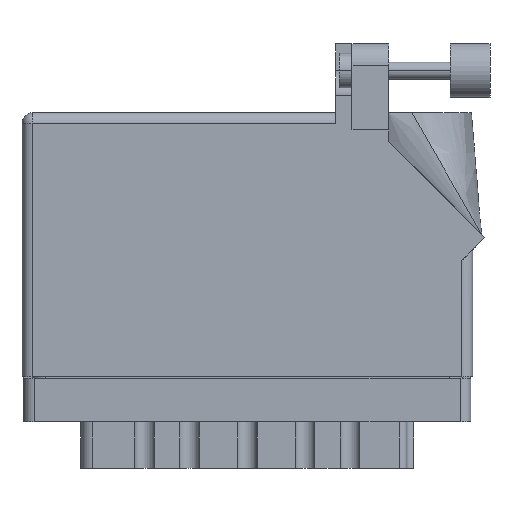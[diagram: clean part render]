
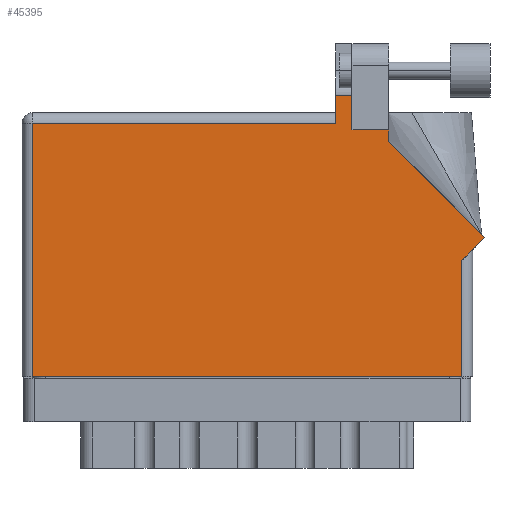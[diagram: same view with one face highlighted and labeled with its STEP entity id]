
A CAD part, front view. The second image highlights one B-rep face of the part: STEP entity #45395.
In plain terms, the highlighted face is planar.
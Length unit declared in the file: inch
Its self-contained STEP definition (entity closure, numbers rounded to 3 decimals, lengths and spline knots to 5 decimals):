
#1114 = CARTESIAN_POINT ( 'NONE',  ( 2.126, 1.43, 0. ) ) ;
#1149 = VERTEX_POINT ( 'NONE', #8238 ) ;
#3136 = VECTOR ( 'NONE', #6639, 39.37008 ) ;
#3262 = CARTESIAN_POINT ( 'NONE',  ( 2.55, 0., 0. ) ) ;
#3443 = ORIENTED_EDGE ( 'NONE', *, *, #29169, .T. ) ;
#3731 = DIRECTION ( 'NONE',  ( 0., 1., 0. ) ) ;
#4015 = CARTESIAN_POINT ( 'NONE',  ( 0., 1.468, 0. ) ) ;
#4046 = VERTEX_POINT ( 'NONE', #38259 ) ;
#4047 = LINE ( 'NONE', #37966, #14964 ) ;
#4328 = VERTEX_POINT ( 'NONE', #36645 ) ;
#4902 = CARTESIAN_POINT ( 'NONE',  ( 1.819, 1.53, 0. ) ) ;
#5037 = FACE_OUTER_BOUND ( 'NONE', #15050, .T. ) ;
#5993 = VERTEX_POINT ( 'NONE', #21692 ) ;
#6279 = DIRECTION ( 'NONE',  ( 0.707, 0.707, 0. ) ) ;
#6639 = DIRECTION ( 'NONE',  ( -1., 0., 0. ) ) ;
#6946 = VERTEX_POINT ( 'NONE', #3262 ) ;
#7095 = CARTESIAN_POINT ( 'NONE',  ( 1.913, 1.43, 0. ) ) ;
#7754 = LINE ( 'NONE', #4015, #37918 ) ;
#7974 = LINE ( 'NONE', #23871, #23864 ) ;
#8238 = CARTESIAN_POINT ( 'NONE',  ( 2.68271, 0.80771, 0. ) ) ;
#8385 = CARTESIAN_POINT ( 'NONE',  ( 2.55, 0.675, 0. ) ) ;
#9418 = ORIENTED_EDGE ( 'NONE', *, *, #36121, .T. ) ;
#9593 = CARTESIAN_POINT ( 'NONE',  ( 2.68271, 0.80771, 0. ) ) ;
#9613 = CARTESIAN_POINT ( 'NONE',  ( 0., 0., 0. ) ) ;
#10214 = CARTESIAN_POINT ( 'NONE',  ( 0.062, 0., 0. ) ) ;
#10884 = VECTOR ( 'NONE', #15582, 39.37008 ) ;
#12349 = EDGE_CURVE ( 'NONE', #29909, #5993, #34075, .T. ) ;
#12456 = ORIENTED_EDGE ( 'NONE', *, *, #20645, .T. ) ;
#12509 = EDGE_CURVE ( 'NONE', #32654, #39599, #7754, .T. ) ;
#13100 = DIRECTION ( 'NONE',  ( 1., 0., 0. ) ) ;
#14572 = DIRECTION ( 'NONE',  ( -1., 0., 0. ) ) ;
#14684 = CARTESIAN_POINT ( 'NONE',  ( 1.819, 1.468, 0. ) ) ;
#14956 = VERTEX_POINT ( 'NONE', #15863 ) ;
#14964 = VECTOR ( 'NONE', #6279, 39.37008 ) ;
#15033 = VERTEX_POINT ( 'NONE', #8385 ) ;
#15050 = EDGE_LOOP ( 'NONE', ( #31628, #37266, #26577, #32310, #3443, #44332, #22404, #15284, #9418, #12456, #29070 ) ) ;
#15099 = LINE ( 'NONE', #9613, #18404 ) ;
#15284 = ORIENTED_EDGE ( 'NONE', *, *, #43805, .T. ) ;
#15582 = DIRECTION ( 'NONE',  ( 0., -1., 0. ) ) ;
#15863 = CARTESIAN_POINT ( 'NONE',  ( 1.819, 1.6315, 0. ) ) ;
#18404 = VECTOR ( 'NONE', #13100, 39.37008 ) ;
#18714 = DIRECTION ( 'NONE',  ( -1., 0., 0. ) ) ;
#18894 = EDGE_CURVE ( 'NONE', #14956, #32654, #38867, .T. ) ;
#18999 = LINE ( 'NONE', #23929, #3136 ) ;
#20383 = CARTESIAN_POINT ( 'NONE',  ( 2.126, 1.36442, 0. ) ) ;
#20645 = EDGE_CURVE ( 'NONE', #4328, #31933, #44143, .T. ) ;
#21097 = VECTOR ( 'NONE', #38250, 39.37008 ) ;
#21474 = VECTOR ( 'NONE', #18714, 39.37008 ) ;
#21692 = CARTESIAN_POINT ( 'NONE',  ( 1.913, 1.6315, 0. ) ) ;
#22404 = ORIENTED_EDGE ( 'NONE', *, *, #24647, .T. ) ;
#23864 = VECTOR ( 'NONE', #27517, 39.37008 ) ;
#23871 = CARTESIAN_POINT ( 'NONE',  ( 2.55, 0.737, 0. ) ) ;
#23929 = CARTESIAN_POINT ( 'NONE',  ( 2.24377, 1.6315, 0. ) ) ;
#23943 = EDGE_CURVE ( 'NONE', #5993, #14956, #18999, .T. ) ;
#24647 = EDGE_CURVE ( 'NONE', #6946, #15033, #7974, .T. ) ;
#24989 = EDGE_CURVE ( 'NONE', #4046, #6946, #15099, .T. ) ;
#26577 = ORIENTED_EDGE ( 'NONE', *, *, #18894, .T. ) ;
#27286 = CARTESIAN_POINT ( 'NONE',  ( 0.062, 1.468, 0. ) ) ;
#27411 = DIRECTION ( 'NONE',  ( 0., 1., 0. ) ) ;
#27517 = DIRECTION ( 'NONE',  ( 0., 1., 0. ) ) ;
#28835 = CARTESIAN_POINT ( 'NONE',  ( 0., 1.53, 0. ) ) ;
#28981 = PLANE ( 'NONE',  #42127 ) ;
#29070 = ORIENTED_EDGE ( 'NONE', *, *, #39798, .T. ) ;
#29169 = EDGE_CURVE ( 'NONE', #39599, #4046, #35932, .T. ) ;
#29909 = VERTEX_POINT ( 'NONE', #7095 ) ;
#31628 = ORIENTED_EDGE ( 'NONE', *, *, #12349, .T. ) ;
#31747 = DIRECTION ( 'NONE',  ( -1., 0., 0. ) ) ;
#31933 = VERTEX_POINT ( 'NONE', #41731 ) ;
#32310 = ORIENTED_EDGE ( 'NONE', *, *, #12509, .T. ) ;
#32654 = VERTEX_POINT ( 'NONE', #14684 ) ;
#34075 = LINE ( 'NONE', #45392, #43956 ) ;
#34088 = DIRECTION ( 'NONE',  ( -0.707, 0.707, 0. ) ) ;
#35452 = DIRECTION ( 'NONE',  ( 0., 0., -1. ) ) ;
#35932 = LINE ( 'NONE', #10214, #21097 ) ;
#36052 = VECTOR ( 'NONE', #34088, 39.37008 ) ;
#36121 = EDGE_CURVE ( 'NONE', #1149, #4328, #45349, .T. ) ;
#36645 = CARTESIAN_POINT ( 'NONE',  ( 2.126, 1.36442, 0. ) ) ;
#37266 = ORIENTED_EDGE ( 'NONE', *, *, #23943, .T. ) ;
#37918 = VECTOR ( 'NONE', #14572, 39.37008 ) ;
#37966 = CARTESIAN_POINT ( 'NONE',  ( 2.612, 0.737, 0. ) ) ;
#38250 = DIRECTION ( 'NONE',  ( 0., -1., 0. ) ) ;
#38259 = CARTESIAN_POINT ( 'NONE',  ( 0.062, 0., 0. ) ) ;
#38867 = LINE ( 'NONE', #4902, #10884 ) ;
#39599 = VERTEX_POINT ( 'NONE', #27286 ) ;
#39798 = EDGE_CURVE ( 'NONE', #31933, #29909, #43923, .T. ) ;
#41731 = CARTESIAN_POINT ( 'NONE',  ( 2.126, 1.43, 0. ) ) ;
#42127 = AXIS2_PLACEMENT_3D ( 'NONE', #28835, #35452, #31747 ) ;
#43805 = EDGE_CURVE ( 'NONE', #15033, #1149, #4047, .T. ) ;
#43923 = LINE ( 'NONE', #1114, #21474 ) ;
#43956 = VECTOR ( 'NONE', #3731, 39.37008 ) ;
#44143 = LINE ( 'NONE', #20383, #44685 ) ;
#44332 = ORIENTED_EDGE ( 'NONE', *, *, #24989, .T. ) ;
#44685 = VECTOR ( 'NONE', #27411, 39.37008 ) ;
#45349 = LINE ( 'NONE', #9593, #36052 ) ;
#45392 = CARTESIAN_POINT ( 'NONE',  ( 1.913, 1.43, 0. ) ) ;
#45395 = ADVANCED_FACE ( 'NONE', ( #5037 ), #28981, .F. ) ;
